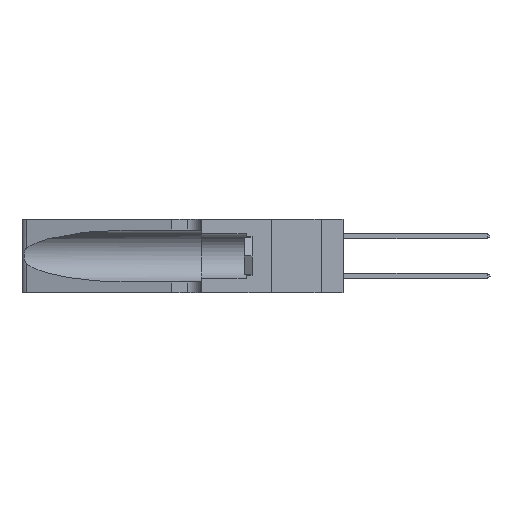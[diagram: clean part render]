
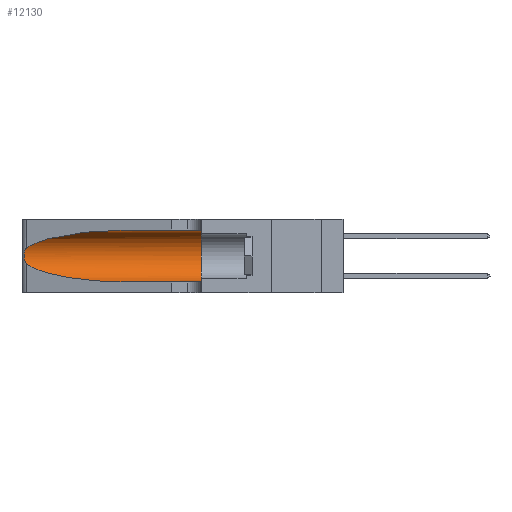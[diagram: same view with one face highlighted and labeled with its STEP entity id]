
A CAD part, left-side view. The second image highlights one B-rep face of the part: STEP entity #12130.
In plain terms, the highlighted cylindrical face has radius 3.308 mm (diameter 6.617 mm), a partial arc.
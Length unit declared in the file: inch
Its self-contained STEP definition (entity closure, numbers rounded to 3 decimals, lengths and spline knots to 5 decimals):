
#467 = EDGE_CURVE ( 'NONE', #9558, #38896, #15088, .T. ) ;
#2314 = CARTESIAN_POINT ( 'NONE',  ( 0.25787, 1.23484, 0.2124 ) ) ;
#3112 = ORIENTED_EDGE ( 'NONE', *, *, #24060, .T. ) ;
#4376 = CARTESIAN_POINT ( 'NONE',  ( 0.25487, 1.22718, 0.22369 ) ) ;
#4611 =( BOUNDED_CURVE ( )  B_SPLINE_CURVE ( 3, ( #15823, #30352, #38448, #4376 ),
 .UNSPECIFIED., .F., .T. ) 
 B_SPLINE_CURVE_WITH_KNOTS ( ( 4, 4 ),
 ( 1.5708, 2.84003 ),
 .UNSPECIFIED. ) 
 CURVE ( )  GEOMETRIC_REPRESENTATION_ITEM ( )  RATIONAL_B_SPLINE_CURVE ( ( 1., 0.87, 0.87, 1. ) ) 
 REPRESENTATION_ITEM ( '' )  );
#5888 = DIRECTION ( 'NONE',  ( 0., -1., 0. ) ) ;
#6825 = VECTOR ( 'NONE', #34233, 39.37008 ) ;
#8804 = CARTESIAN_POINT ( 'NONE',  ( 0.26075, 1.23896, 0.178 ) ) ;
#8942 = CARTESIAN_POINT ( 'NONE',  ( 0.25639, 1.23186, 0.15144 ) ) ;
#9051 = CARTESIAN_POINT ( 'NONE',  ( 0.1305, 0.72297, 0.31525 ) ) ;
#9207 = CARTESIAN_POINT ( 'NONE',  ( 0.25789, 1.23486, 0.15765 ) ) ;
#9558 = VERTEX_POINT ( 'NONE', #10284 ) ;
#10284 = CARTESIAN_POINT ( 'NONE',  ( 0.1305, 0.35, 0.31525 ) ) ;
#11149 = EDGE_CURVE ( 'NONE', #14353, #17253, #24531, .T. ) ;
#12092 = VERTEX_POINT ( 'NONE', #32524 ) ;
#12110 = EDGE_CURVE ( 'NONE', #17253, #12092, #35945, .T. ) ;
#12130 = ADVANCED_FACE ( 'NONE', ( #20717 ), #29951, .F. ) ;
#12476 = CARTESIAN_POINT ( 'NONE',  ( 0.26018, 1.23835, 0.19895 ) ) ;
#12668 = AXIS2_PLACEMENT_3D ( 'NONE', #20813, #30186, #40028 ) ;
#14353 = VERTEX_POINT ( 'NONE', #26262 ) ;
#14454 = LINE ( 'NONE', #26950, #38810 ) ;
#14660 = ORIENTED_EDGE ( 'NONE', *, *, #38056, .F. ) ;
#15050 = CARTESIAN_POINT ( 'NONE',  ( 0.26017, 1.23833, 0.17102 ) ) ;
#15088 = CIRCLE ( 'NONE', #12668, 0.13025 ) ;
#15823 = CARTESIAN_POINT ( 'NONE',  ( 0.1305, 0.72297, 0.31525 ) ) ;
#16376 = DIRECTION ( 'NONE',  ( 0., -1., 0. ) ) ;
#17176 = EDGE_CURVE ( 'NONE', #18183, #14353, #4611, .T. ) ;
#17253 = VERTEX_POINT ( 'NONE', #28252 ) ;
#17879 = CARTESIAN_POINT ( 'NONE',  ( 0.25854, 1.2359, 0.20912 ) ) ;
#18183 = VERTEX_POINT ( 'NONE', #9051 ) ;
#18656 = CARTESIAN_POINT ( 'NONE',  ( 0.1305, 1.61858, 0.05475 ) ) ;
#18863 = ORIENTED_EDGE ( 'NONE', *, *, #467, .F. ) ;
#19430 = AXIS2_PLACEMENT_3D ( 'NONE', #34978, #16376, #32018 ) ;
#20717 = FACE_OUTER_BOUND ( 'NONE', #36011, .T. ) ;
#20813 = CARTESIAN_POINT ( 'NONE',  ( 0.1305, 0.35, 0.185 ) ) ;
#20919 = CARTESIAN_POINT ( 'NONE',  ( 0.25639, 1.23184, 0.21858 ) ) ;
#22650 = CARTESIAN_POINT ( 'NONE',  ( 0.18966, 0.96281, 0.05475 ) ) ;
#22804 = CARTESIAN_POINT ( 'NONE',  ( 0.2373, 1.15595, 0.08982 ) ) ;
#23917 = CARTESIAN_POINT ( 'NONE',  ( 0.25487, 1.22718, 0.22369 ) ) ;
#24060 = EDGE_CURVE ( 'NONE', #12092, #38896, #29696, .T. ) ;
#24531 = B_SPLINE_CURVE_WITH_KNOTS ( 'NONE', 3,
 ( #23917, #36493, #20919, #2314, #17879, #12476, #27839, #8804, #15050, #30819, #9207, #8942, #30678, #37183 ),
 .UNSPECIFIED., .F., .F.,
 ( 4, 2, 2, 2, 2, 2, 4 ),
 ( 0., 0.00027, 0.00053, 0.00107, 0.0016, 0.00187, 0.00214 ),
 .UNSPECIFIED. ) ;
#26262 = CARTESIAN_POINT ( 'NONE',  ( 0.25487, 1.22718, 0.22369 ) ) ;
#26950 = CARTESIAN_POINT ( 'NONE',  ( 0.1305, 1.61858, 0.31525 ) ) ;
#27839 = CARTESIAN_POINT ( 'NONE',  ( 0.26075, 1.23896, 0.19203 ) ) ;
#27976 = CARTESIAN_POINT ( 'NONE',  ( 0.1305, 0.35, 0.05475 ) ) ;
#28252 = CARTESIAN_POINT ( 'NONE',  ( 0.25487, 1.22718, 0.14631 ) ) ;
#29249 = ORIENTED_EDGE ( 'NONE', *, *, #12110, .T. ) ;
#29696 = LINE ( 'NONE', #18656, #6825 ) ;
#29951 = CYLINDRICAL_SURFACE ( 'NONE', #19430, 0.13025 ) ;
#30186 = DIRECTION ( 'NONE',  ( 0., 1., 0. ) ) ;
#30352 = CARTESIAN_POINT ( 'NONE',  ( 0.18966, 0.96281, 0.31525 ) ) ;
#30678 = CARTESIAN_POINT ( 'NONE',  ( 0.25555, 1.22993, 0.14849 ) ) ;
#30819 = CARTESIAN_POINT ( 'NONE',  ( 0.25856, 1.23593, 0.16098 ) ) ;
#31262 = ORIENTED_EDGE ( 'NONE', *, *, #11149, .T. ) ;
#32018 = DIRECTION ( 'NONE',  ( 0., 0., -1. ) ) ;
#32524 = CARTESIAN_POINT ( 'NONE',  ( 0.1305, 0.72297, 0.05475 ) ) ;
#32554 = CARTESIAN_POINT ( 'NONE',  ( 0.1305, 0.72297, 0.05475 ) ) ;
#34233 = DIRECTION ( 'NONE',  ( 0., -1., 0. ) ) ;
#34978 = CARTESIAN_POINT ( 'NONE',  ( 0.1305, 1.61858, 0.185 ) ) ;
#35012 = ORIENTED_EDGE ( 'NONE', *, *, #17176, .T. ) ;
#35113 = CARTESIAN_POINT ( 'NONE',  ( 0.25487, 1.22718, 0.14631 ) ) ;
#35945 =( BOUNDED_CURVE ( )  B_SPLINE_CURVE ( 3, ( #35113, #22804, #22650, #32554 ),
 .UNSPECIFIED., .F., .F. ) 
 B_SPLINE_CURVE_WITH_KNOTS ( ( 4, 4 ),
 ( 3.44316, 4.71239 ),
 .UNSPECIFIED. ) 
 CURVE ( )  GEOMETRIC_REPRESENTATION_ITEM ( )  RATIONAL_B_SPLINE_CURVE ( ( 1., 0.87, 0.87, 1. ) ) 
 REPRESENTATION_ITEM ( '' )  );
#36011 = EDGE_LOOP ( 'NONE', ( #35012, #31262, #29249, #3112, #18863, #14660 ) ) ;
#36493 = CARTESIAN_POINT ( 'NONE',  ( 0.25555, 1.22994, 0.2215 ) ) ;
#37183 = CARTESIAN_POINT ( 'NONE',  ( 0.25487, 1.22718, 0.14631 ) ) ;
#38056 = EDGE_CURVE ( 'NONE', #18183, #9558, #14454, .T. ) ;
#38448 = CARTESIAN_POINT ( 'NONE',  ( 0.2373, 1.15595, 0.28018 ) ) ;
#38810 = VECTOR ( 'NONE', #5888, 39.37008 ) ;
#38896 = VERTEX_POINT ( 'NONE', #27976 ) ;
#40028 = DIRECTION ( 'NONE',  ( 0., 0., 1. ) ) ;
